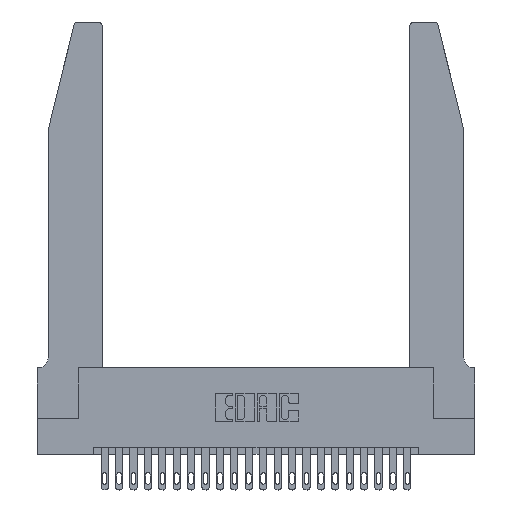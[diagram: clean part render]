
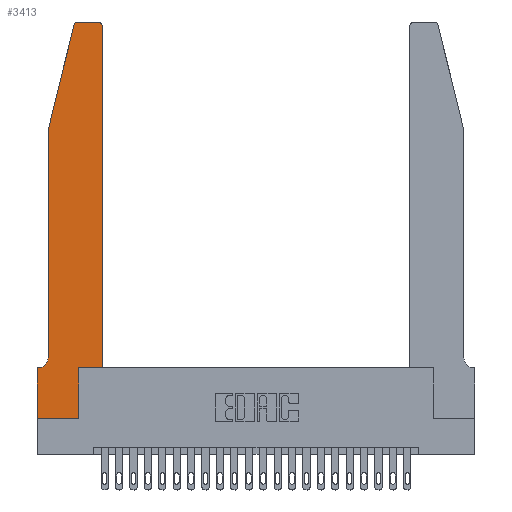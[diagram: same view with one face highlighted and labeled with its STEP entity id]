
A CAD part, top view. The second image highlights one B-rep face of the part: STEP entity #3413.
In plain terms, the highlighted planar face has unit normal (0, 0, 1).
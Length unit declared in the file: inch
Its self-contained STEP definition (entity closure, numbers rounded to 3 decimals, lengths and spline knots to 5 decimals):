
#40 = DIRECTION ( 'NONE',  ( 0., 0., 1. ) ) ;
#380 = EDGE_CURVE ( 'NONE', #12975, #2061, #23252, .T. ) ;
#461 = VERTEX_POINT ( 'NONE', #7186 ) ;
#508 = VECTOR ( 'NONE', #16770, 39.37008 ) ;
#851 = LINE ( 'NONE', #11296, #23754 ) ;
#901 = EDGE_CURVE ( 'NONE', #21938, #461, #11577, .T. ) ;
#1027 = CARTESIAN_POINT ( 'NONE',  ( 0.2865, 0.35, 0.37 ) ) ;
#1222 = EDGE_CURVE ( 'NONE', #10616, #7645, #18403, .T. ) ;
#1279 = DIRECTION ( 'NONE',  ( -1., 0., 0. ) ) ;
#1680 = VERTEX_POINT ( 'NONE', #2476 ) ;
#1693 = ORIENTED_EDGE ( 'NONE', *, *, #6521, .T. ) ;
#1698 = ORIENTED_EDGE ( 'NONE', *, *, #8259, .T. ) ;
#1863 = CARTESIAN_POINT ( 'NONE',  ( 0.2865, 0., 0.37 ) ) ;
#2061 = VERTEX_POINT ( 'NONE', #12076 ) ;
#2476 = CARTESIAN_POINT ( 'NONE',  ( 0.284, 2.75, 0.37 ) ) ;
#2544 = DIRECTION ( 'NONE',  ( -1., 0., 0. ) ) ;
#2835 = EDGE_CURVE ( 'NONE', #7718, #1680, #6495, .T. ) ;
#3131 = DIRECTION ( 'NONE',  ( 1., 0., 0. ) ) ;
#3275 = CARTESIAN_POINT ( 'NONE',  ( 0.2605, 2.75, 0.37 ) ) ;
#3413 = ADVANCED_FACE ( 'NONE', ( #15939 ), #21001, .T. ) ;
#3508 = CARTESIAN_POINT ( 'NONE',  ( 0.4505, 0.35, 0.37 ) ) ;
#3998 = CARTESIAN_POINT ( 'NONE',  ( 0., 0.35, 0.37 ) ) ;
#4598 = VERTEX_POINT ( 'NONE', #1863 ) ;
#4966 = ORIENTED_EDGE ( 'NONE', *, *, #20992, .T. ) ;
#5575 = LINE ( 'NONE', #3508, #508 ) ;
#5822 = DIRECTION ( 'NONE',  ( 1., 0., 0. ) ) ;
#6495 = LINE ( 'NONE', #3275, #10903 ) ;
#6521 = EDGE_CURVE ( 'NONE', #4598, #10473, #6588, .T. ) ;
#6588 = LINE ( 'NONE', #1027, #20552 ) ;
#6731 = CARTESIAN_POINT ( 'NONE',  ( 0., 0., 0.37 ) ) ;
#6977 = CARTESIAN_POINT ( 'NONE',  ( 0., 0., 0.37 ) ) ;
#7186 = CARTESIAN_POINT ( 'NONE',  ( 0.0055, 0.35, 0.37 ) ) ;
#7302 = DIRECTION ( 'NONE',  ( 0., -1., 0. ) ) ;
#7456 = DIRECTION ( 'NONE',  ( -1., 0., 0. ) ) ;
#7645 = VERTEX_POINT ( 'NONE', #17441 ) ;
#7718 = VERTEX_POINT ( 'NONE', #20695 ) ;
#8259 = EDGE_CURVE ( 'NONE', #2061, #21938, #16315, .T. ) ;
#8378 = CARTESIAN_POINT ( 'NONE',  ( 0.4505, 0.35, 0.37 ) ) ;
#8763 = ORIENTED_EDGE ( 'NONE', *, *, #20233, .T. ) ;
#9348 = CARTESIAN_POINT ( 'NONE',  ( 0.2865, 0.35, 0.37 ) ) ;
#9361 = DIRECTION ( 'NONE',  ( 0., 0., 1. ) ) ;
#9428 = CARTESIAN_POINT ( 'NONE',  ( 0., 0.35, 0.37 ) ) ;
#9467 = VECTOR ( 'NONE', #10290, 39.37008 ) ;
#9716 = AXIS2_PLACEMENT_3D ( 'NONE', #9428, #40, #11181 ) ;
#9939 = EDGE_CURVE ( 'NONE', #17114, #4598, #851, .T. ) ;
#10290 = DIRECTION ( 'NONE',  ( 0., 1., 0. ) ) ;
#10473 = VERTEX_POINT ( 'NONE', #9348 ) ;
#10616 = VERTEX_POINT ( 'NONE', #20577 ) ;
#10903 = VECTOR ( 'NONE', #1279, 39.37008 ) ;
#10997 = ORIENTED_EDGE ( 'NONE', *, *, #2835, .T. ) ;
#11181 = DIRECTION ( 'NONE',  ( 1., 0., 0. ) ) ;
#11256 = LINE ( 'NONE', #21337, #21709 ) ;
#11296 = CARTESIAN_POINT ( 'NONE',  ( 0., 0., 0.37 ) ) ;
#11567 = VERTEX_POINT ( 'NONE', #3998 ) ;
#11577 = CIRCLE ( 'NONE', #19909, 0.07 ) ;
#11913 = VECTOR ( 'NONE', #16814, 39.37008 ) ;
#12076 = CARTESIAN_POINT ( 'NONE',  ( 0.0755, 2., 0.37 ) ) ;
#12141 = CARTESIAN_POINT ( 'NONE',  ( 0.0755, 0.42, 0.37 ) ) ;
#12975 = VERTEX_POINT ( 'NONE', #18245 ) ;
#13096 = CARTESIAN_POINT ( 'NONE',  ( 0.0055, 0.42, 0.37 ) ) ;
#13130 = EDGE_LOOP ( 'NONE', ( #10997, #8763, #15589, #1698, #14351, #4966, #23051, #14217, #1693, #20498, #13504, #16363 ) ) ;
#13504 = ORIENTED_EDGE ( 'NONE', *, *, #1222, .T. ) ;
#14217 = ORIENTED_EDGE ( 'NONE', *, *, #9939, .T. ) ;
#14351 = ORIENTED_EDGE ( 'NONE', *, *, #901, .T. ) ;
#14816 = EDGE_CURVE ( 'NONE', #7645, #7718, #17920, .T. ) ;
#15589 = ORIENTED_EDGE ( 'NONE', *, *, #380, .T. ) ;
#15939 = FACE_OUTER_BOUND ( 'NONE', #13130, .T. ) ;
#16315 = LINE ( 'NONE', #17483, #16591 ) ;
#16363 = ORIENTED_EDGE ( 'NONE', *, *, #14816, .T. ) ;
#16591 = VECTOR ( 'NONE', #7302, 39.37008 ) ;
#16770 = DIRECTION ( 'NONE',  ( 1., 0., 0. ) ) ;
#16814 = DIRECTION ( 'NONE',  ( -0.239, -0.971, 0. ) ) ;
#16886 = AXIS2_PLACEMENT_3D ( 'NONE', #22335, #24313, #3131 ) ;
#17114 = VERTEX_POINT ( 'NONE', #6977 ) ;
#17441 = CARTESIAN_POINT ( 'NONE',  ( 0.4505, 2.72, 0.37 ) ) ;
#17483 = CARTESIAN_POINT ( 'NONE',  ( 0.0755, 2., 0.37 ) ) ;
#17499 = EDGE_CURVE ( 'NONE', #11567, #17114, #22550, .T. ) ;
#17693 = DIRECTION ( 'NONE',  ( 0., -1., 0. ) ) ;
#17920 = CIRCLE ( 'NONE', #16886, 0.03 ) ;
#18245 = CARTESIAN_POINT ( 'NONE',  ( 0.25487, 2.72718, 0.37 ) ) ;
#18298 = DIRECTION ( 'NONE',  ( 0., 1., 0. ) ) ;
#18403 = LINE ( 'NONE', #8378, #9467 ) ;
#18716 = AXIS2_PLACEMENT_3D ( 'NONE', #20864, #9361, #18954 ) ;
#18853 = DIRECTION ( 'NONE',  ( 0., 0., -1. ) ) ;
#18954 = DIRECTION ( 'NONE',  ( 1., 0., 0. ) ) ;
#19909 = AXIS2_PLACEMENT_3D ( 'NONE', #13096, #18853, #7456 ) ;
#20233 = EDGE_CURVE ( 'NONE', #1680, #12975, #22583, .T. ) ;
#20498 = ORIENTED_EDGE ( 'NONE', *, *, #22260, .T. ) ;
#20552 = VECTOR ( 'NONE', #18298, 39.37008 ) ;
#20577 = CARTESIAN_POINT ( 'NONE',  ( 0.4505, 0.35, 0.37 ) ) ;
#20695 = CARTESIAN_POINT ( 'NONE',  ( 0.4205, 2.75, 0.37 ) ) ;
#20864 = CARTESIAN_POINT ( 'NONE',  ( 0.284, 2.72, 0.37 ) ) ;
#20992 = EDGE_CURVE ( 'NONE', #461, #11567, #11256, .T. ) ;
#21001 = PLANE ( 'NONE',  #9716 ) ;
#21337 = CARTESIAN_POINT ( 'NONE',  ( 0.0755, 0.35, 0.37 ) ) ;
#21709 = VECTOR ( 'NONE', #2544, 39.37008 ) ;
#21938 = VERTEX_POINT ( 'NONE', #12141 ) ;
#22260 = EDGE_CURVE ( 'NONE', #10473, #10616, #5575, .T. ) ;
#22335 = CARTESIAN_POINT ( 'NONE',  ( 0.4205, 2.72, 0.37 ) ) ;
#22411 = CARTESIAN_POINT ( 'NONE',  ( 0.0755, 2., 0.37 ) ) ;
#22550 = LINE ( 'NONE', #6731, #23745 ) ;
#22583 = CIRCLE ( 'NONE', #18716, 0.03 ) ;
#23051 = ORIENTED_EDGE ( 'NONE', *, *, #17499, .T. ) ;
#23252 = LINE ( 'NONE', #22411, #11913 ) ;
#23745 = VECTOR ( 'NONE', #17693, 39.37008 ) ;
#23754 = VECTOR ( 'NONE', #5822, 39.37008 ) ;
#24313 = DIRECTION ( 'NONE',  ( 0., 0., 1. ) ) ;
